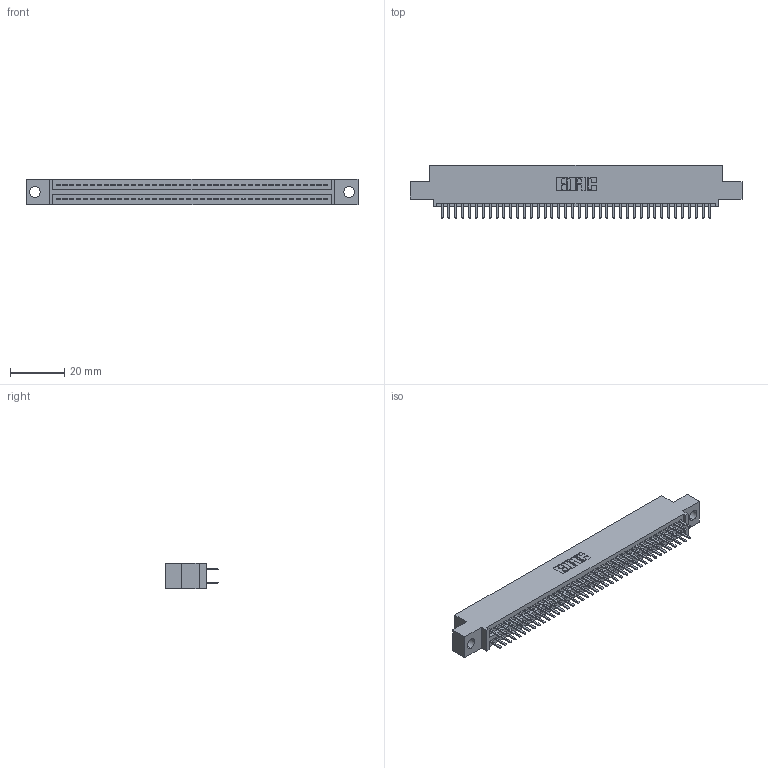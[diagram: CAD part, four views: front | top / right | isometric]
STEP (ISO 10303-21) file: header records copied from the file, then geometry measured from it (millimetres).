
FILE_DESCRIPTION (( 'STEP AP203' ), '1' );
FILE_NAME ('395-080-520-504.STEP', '2021-06-17T06:56:38', ( '' ), ( '' ), 'SwSTEP 2.0', 'SolidWorks 2020', '' );
FILE_SCHEMA (( 'CONFIG_CONTROL_DESIGN' ));
Length unit declared in the file: inch
Products named in the file (3): 345-292-001_345-293-120; 395-080-520-504; 345 Part_0.110 Offset - 0.156 Dia-TI
Assembly tree (81 placements, depth 2):
  395-080-520-504
    345 Part_0.110 Offset - 0.156 Dia-TI
    345-292-001_345-293-120  x80
Bounding box: 122.81 x 19.68 x 9.4 mm (x, y, z)
Volume: 11696.7 mm3; surface area: 17120.6 mm2
Topology: 81 solids, 81 shells, 4464 faces, 12949 edges, 8418 vertices
Faces by surface type: plane 2898, cylinder 1566
Entity records: 32319 total; most frequent: CARTESIAN_POINT 5438, ORIENTED_EDGE 5358, DIRECTION 4783, EDGE_CURVE 2679, LINE 2383, VECTOR 2383, VERTEX_POINT 1782, AXIS2_PLACEMENT_3D 1200
